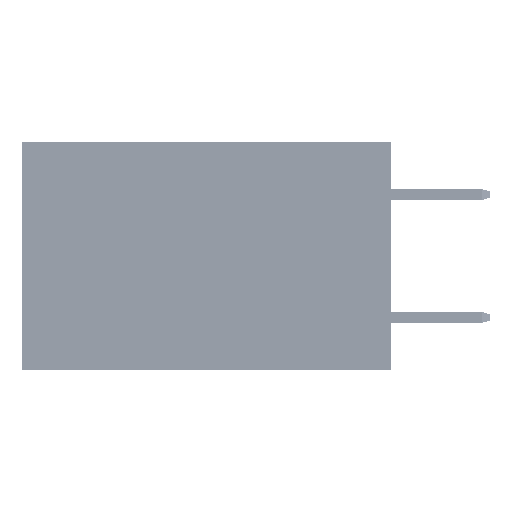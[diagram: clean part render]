
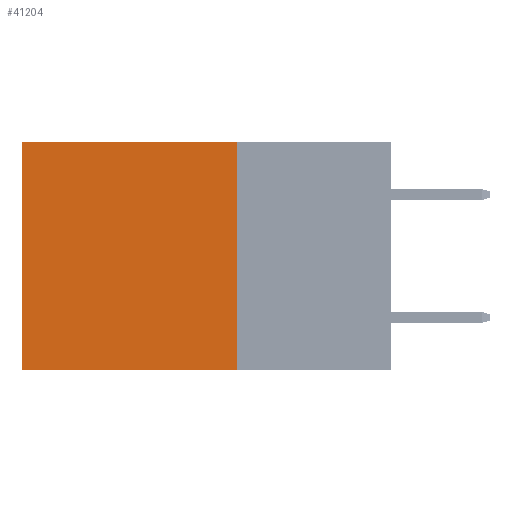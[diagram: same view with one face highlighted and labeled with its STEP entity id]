
A CAD part, left-side view. The second image highlights one B-rep face of the part: STEP entity #41204.
In plain terms, the highlighted planar face has unit normal (-1, 0, 0).
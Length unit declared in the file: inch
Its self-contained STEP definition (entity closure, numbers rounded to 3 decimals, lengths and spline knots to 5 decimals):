
#1440 = AXIS2_PLACEMENT_3D ( 'NONE', #7406, #34961, #11857 ) ;
#3616 = EDGE_CURVE ( 'NONE', #14205, #21423, #33024, .T. ) ;
#5036 = VECTOR ( 'NONE', #38968, 39.37008 ) ;
#5607 = VERTEX_POINT ( 'NONE', #6270 ) ;
#6270 = CARTESIAN_POINT ( 'NONE',  ( 0.2875, 0.6, -0.37 ) ) ;
#7406 = CARTESIAN_POINT ( 'NONE',  ( 0.2875, 0.25, 0. ) ) ;
#9055 = CARTESIAN_POINT ( 'NONE',  ( 0.2875, 0.6, 0. ) ) ;
#9070 = EDGE_CURVE ( 'NONE', #14205, #15047, #9811, .T. ) ;
#9551 = CARTESIAN_POINT ( 'NONE',  ( 0.2875, 0.25, -0.37 ) ) ;
#9811 = LINE ( 'NONE', #24305, #34910 ) ;
#11857 = DIRECTION ( 'NONE',  ( 0., 0., -1. ) ) ;
#14205 = VERTEX_POINT ( 'NONE', #45151 ) ;
#14581 = CARTESIAN_POINT ( 'NONE',  ( 0.2875, 0.25, 0. ) ) ;
#15047 = VERTEX_POINT ( 'NONE', #15328 ) ;
#15328 = CARTESIAN_POINT ( 'NONE',  ( 0.2875, 0.6, 0. ) ) ;
#19166 = EDGE_CURVE ( 'NONE', #15047, #5607, #35543, .T. ) ;
#19789 = ORIENTED_EDGE ( 'NONE', *, *, #40484, .F. ) ;
#19997 = EDGE_LOOP ( 'NONE', ( #36698, #19789, #22707, #44435 ) ) ;
#21423 = VERTEX_POINT ( 'NONE', #9551 ) ;
#22707 = ORIENTED_EDGE ( 'NONE', *, *, #3616, .F. ) ;
#24305 = CARTESIAN_POINT ( 'NONE',  ( 0.2875, 0.25, 0. ) ) ;
#27748 = DIRECTION ( 'NONE',  ( 0., 1., 0. ) ) ;
#32565 = FACE_OUTER_BOUND ( 'NONE', #19997, .T. ) ;
#33024 = LINE ( 'NONE', #14581, #40987 ) ;
#34910 = VECTOR ( 'NONE', #27748, 39.37008 ) ;
#34961 = DIRECTION ( 'NONE',  ( 1., 0., 0. ) ) ;
#35543 = LINE ( 'NONE', #9055, #50160 ) ;
#36289 = LINE ( 'NONE', #50025, #5036 ) ;
#36698 = ORIENTED_EDGE ( 'NONE', *, *, #19166, .T. ) ;
#38968 = DIRECTION ( 'NONE',  ( 0., 1., 0. ) ) ;
#40484 = EDGE_CURVE ( 'NONE', #21423, #5607, #36289, .T. ) ;
#40987 = VECTOR ( 'NONE', #41942, 39.37008 ) ;
#41204 = ADVANCED_FACE ( 'NONE', ( #32565 ), #47072, .F. ) ;
#41942 = DIRECTION ( 'NONE',  ( 0., 0., -1. ) ) ;
#44435 = ORIENTED_EDGE ( 'NONE', *, *, #9070, .T. ) ;
#45151 = CARTESIAN_POINT ( 'NONE',  ( 0.2875, 0.25, 0. ) ) ;
#47072 = PLANE ( 'NONE',  #1440 ) ;
#48376 = DIRECTION ( 'NONE',  ( 0., 0., -1. ) ) ;
#50025 = CARTESIAN_POINT ( 'NONE',  ( 0.2875, 0.25, -0.37 ) ) ;
#50160 = VECTOR ( 'NONE', #48376, 39.37008 ) ;
